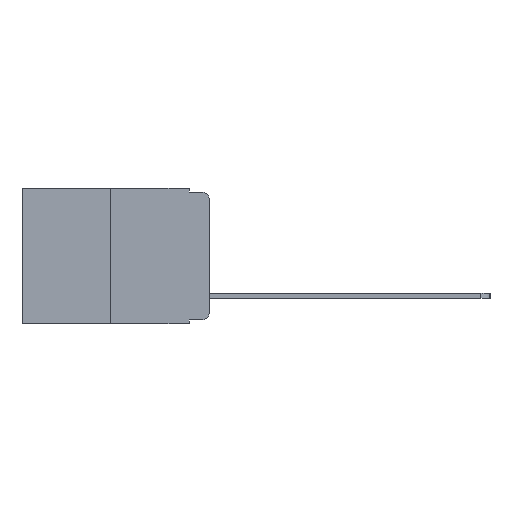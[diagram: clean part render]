
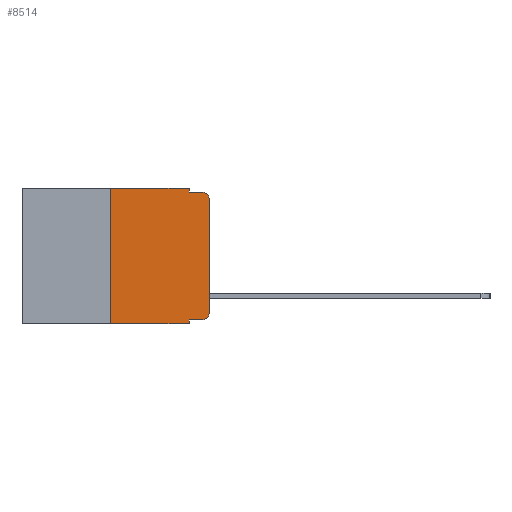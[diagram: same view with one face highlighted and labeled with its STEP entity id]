
A CAD part, left-side view. The second image highlights one B-rep face of the part: STEP entity #8514.
In plain terms, the highlighted planar face has unit normal (-1, 0, 0).
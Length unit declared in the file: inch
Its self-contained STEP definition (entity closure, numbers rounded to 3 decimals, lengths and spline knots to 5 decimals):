
#221 = EDGE_CURVE ( 'NONE', #878, #2521, #5313, .T. ) ;
#263 = VECTOR ( 'NONE', #12168, 39.37008 ) ;
#268 = DIRECTION ( 'NONE',  ( 0., 0., 1. ) ) ;
#473 = CARTESIAN_POINT ( 'NONE',  ( 0., 0.051, -0.01 ) ) ;
#602 = VERTEX_POINT ( 'NONE', #7928 ) ;
#878 = VERTEX_POINT ( 'NONE', #3494 ) ;
#882 = VERTEX_POINT ( 'NONE', #1521 ) ;
#1121 = LINE ( 'NONE', #2599, #10690 ) ;
#1375 = EDGE_CURVE ( 'NONE', #3216, #602, #12333, .T. ) ;
#1515 = DIRECTION ( 'NONE',  ( 0., -1., 0. ) ) ;
#1521 = CARTESIAN_POINT ( 'NONE',  ( 0., 0.051, -0.333 ) ) ;
#1569 = LINE ( 'NONE', #5606, #8675 ) ;
#1629 = PLANE ( 'NONE',  #12232 ) ;
#1755 = ORIENTED_EDGE ( 'NONE', *, *, #1375, .T. ) ;
#1776 = VERTEX_POINT ( 'NONE', #2062 ) ;
#2038 = EDGE_CURVE ( 'NONE', #882, #3216, #10302, .T. ) ;
#2062 = CARTESIAN_POINT ( 'NONE',  ( 0., 0.02, -0.01 ) ) ;
#2177 = AXIS2_PLACEMENT_3D ( 'NONE', #2771, #9441, #3800 ) ;
#2211 = CARTESIAN_POINT ( 'NONE',  ( 0., 0.25, -0.343 ) ) ;
#2521 = VERTEX_POINT ( 'NONE', #11808 ) ;
#2597 = ORIENTED_EDGE ( 'NONE', *, *, #8503, .F. ) ;
#2599 = CARTESIAN_POINT ( 'NONE',  ( 0., 0.051, 0. ) ) ;
#2631 = EDGE_CURVE ( 'NONE', #6512, #5852, #8564, .T. ) ;
#2771 = CARTESIAN_POINT ( 'NONE',  ( 0., 0.02, -0.03 ) ) ;
#2976 = ORIENTED_EDGE ( 'NONE', *, *, #5998, .F. ) ;
#2994 = VECTOR ( 'NONE', #6255, 39.37008 ) ;
#3216 = VERTEX_POINT ( 'NONE', #3338 ) ;
#3338 = CARTESIAN_POINT ( 'NONE',  ( 0., 0.02, -0.333 ) ) ;
#3386 = EDGE_CURVE ( 'NONE', #882, #5852, #5907, .T. ) ;
#3420 = DIRECTION ( 'NONE',  ( 0., 0., -1. ) ) ;
#3494 = CARTESIAN_POINT ( 'NONE',  ( 0., 0.25, 0. ) ) ;
#3616 = FACE_OUTER_BOUND ( 'NONE', #6580, .T. ) ;
#3618 = DIRECTION ( 'NONE',  ( 0., 0., -1. ) ) ;
#3800 = DIRECTION ( 'NONE',  ( 0., 0., -1. ) ) ;
#4164 = CARTESIAN_POINT ( 'NONE',  ( 0., 0.051, -0.343 ) ) ;
#4670 = DIRECTION ( 'NONE',  ( 0., 0., -1. ) ) ;
#4715 = CARTESIAN_POINT ( 'NONE',  ( 0., 0., 0. ) ) ;
#4813 = CIRCLE ( 'NONE', #2177, 0.02 ) ;
#5218 = ORIENTED_EDGE ( 'NONE', *, *, #9724, .T. ) ;
#5313 = LINE ( 'NONE', #9071, #2994 ) ;
#5506 = CARTESIAN_POINT ( 'NONE',  ( 0., 0.051, -0.333 ) ) ;
#5606 = CARTESIAN_POINT ( 'NONE',  ( 0., 0.051, -0.01 ) ) ;
#5852 = VERTEX_POINT ( 'NONE', #4164 ) ;
#5907 = LINE ( 'NONE', #8478, #263 ) ;
#5998 = EDGE_CURVE ( 'NONE', #6512, #878, #6001, .T. ) ;
#6001 = LINE ( 'NONE', #7212, #10635 ) ;
#6255 = DIRECTION ( 'NONE',  ( 0., -1., 0. ) ) ;
#6512 = VERTEX_POINT ( 'NONE', #2211 ) ;
#6563 = DIRECTION ( 'NONE',  ( 0., -1., 0. ) ) ;
#6580 = EDGE_LOOP ( 'NONE', ( #10019, #5218, #2597, #11636, #11485, #2976, #10799, #7930, #6908, #1755 ) ) ;
#6679 = VERTEX_POINT ( 'NONE', #8249 ) ;
#6882 = VECTOR ( 'NONE', #10318, 39.37008 ) ;
#6908 = ORIENTED_EDGE ( 'NONE', *, *, #2038, .T. ) ;
#7212 = CARTESIAN_POINT ( 'NONE',  ( 0., 0.25, 0. ) ) ;
#7876 = EDGE_CURVE ( 'NONE', #2521, #8420, #1121, .T. ) ;
#7928 = CARTESIAN_POINT ( 'NONE',  ( 0., 0., -0.313 ) ) ;
#7930 = ORIENTED_EDGE ( 'NONE', *, *, #3386, .F. ) ;
#8249 = CARTESIAN_POINT ( 'NONE',  ( 0., 0., -0.03 ) ) ;
#8420 = VERTEX_POINT ( 'NONE', #473 ) ;
#8429 = CARTESIAN_POINT ( 'NONE',  ( 0., 0.473, 0. ) ) ;
#8478 = CARTESIAN_POINT ( 'NONE',  ( 0., 0.051, 0. ) ) ;
#8503 = EDGE_CURVE ( 'NONE', #8420, #1776, #1569, .T. ) ;
#8514 = ADVANCED_FACE ( 'NONE', ( #3616 ), #1629, .F. ) ;
#8564 = LINE ( 'NONE', #10082, #10988 ) ;
#8675 = VECTOR ( 'NONE', #6563, 39.37008 ) ;
#9071 = CARTESIAN_POINT ( 'NONE',  ( 0., 0.473, 0. ) ) ;
#9111 = DIRECTION ( 'NONE',  ( -1., 0., 0. ) ) ;
#9250 = DIRECTION ( 'NONE',  ( 0., -1., 0. ) ) ;
#9331 = LINE ( 'NONE', #4715, #6882 ) ;
#9441 = DIRECTION ( 'NONE',  ( -1., 0., 0. ) ) ;
#9488 = AXIS2_PLACEMENT_3D ( 'NONE', #10855, #9111, #3420 ) ;
#9724 = EDGE_CURVE ( 'NONE', #6679, #1776, #4813, .T. ) ;
#10004 = VECTOR ( 'NONE', #9250, 39.37008 ) ;
#10019 = ORIENTED_EDGE ( 'NONE', *, *, #10353, .T. ) ;
#10082 = CARTESIAN_POINT ( 'NONE',  ( 0., 0.473, -0.343 ) ) ;
#10276 = DIRECTION ( 'NONE',  ( 1., 0., 0. ) ) ;
#10302 = LINE ( 'NONE', #5506, #10004 ) ;
#10318 = DIRECTION ( 'NONE',  ( 0., 0., 1. ) ) ;
#10353 = EDGE_CURVE ( 'NONE', #602, #6679, #9331, .T. ) ;
#10635 = VECTOR ( 'NONE', #268, 39.37008 ) ;
#10690 = VECTOR ( 'NONE', #3618, 39.37008 ) ;
#10799 = ORIENTED_EDGE ( 'NONE', *, *, #2631, .T. ) ;
#10855 = CARTESIAN_POINT ( 'NONE',  ( 0., 0.02, -0.313 ) ) ;
#10988 = VECTOR ( 'NONE', #1515, 39.37008 ) ;
#11485 = ORIENTED_EDGE ( 'NONE', *, *, #221, .F. ) ;
#11636 = ORIENTED_EDGE ( 'NONE', *, *, #7876, .F. ) ;
#11808 = CARTESIAN_POINT ( 'NONE',  ( 0., 0.051, 0. ) ) ;
#12168 = DIRECTION ( 'NONE',  ( 0., 0., -1. ) ) ;
#12232 = AXIS2_PLACEMENT_3D ( 'NONE', #8429, #10276, #4670 ) ;
#12333 = CIRCLE ( 'NONE', #9488, 0.02 ) ;
